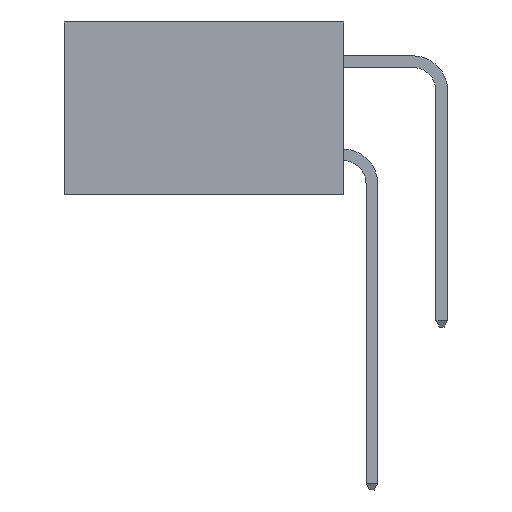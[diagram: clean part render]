
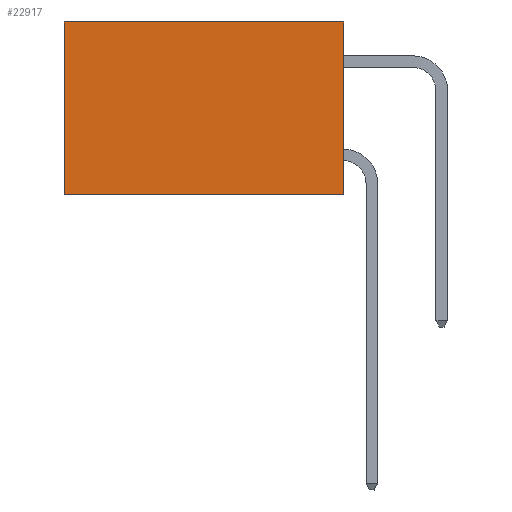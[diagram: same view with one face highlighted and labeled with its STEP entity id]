
A CAD part, left-side view. The second image highlights one B-rep face of the part: STEP entity #22917.
In plain terms, the highlighted planar face has unit normal (-1, 0, 0).
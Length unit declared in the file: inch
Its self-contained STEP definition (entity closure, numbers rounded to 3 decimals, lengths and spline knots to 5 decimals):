
#983 = VECTOR ( 'NONE', #11977, 39.37008 ) ;
#1222 = VERTEX_POINT ( 'NONE', #29377 ) ;
#1296 = VERTEX_POINT ( 'NONE', #10674 ) ;
#2550 = DIRECTION ( 'NONE',  ( 0., 0., -1. ) ) ;
#4002 = LINE ( 'NONE', #14784, #24245 ) ;
#4293 = ORIENTED_EDGE ( 'NONE', *, *, #30141, .T. ) ;
#5652 = DIRECTION ( 'NONE',  ( 0., 1., 0. ) ) ;
#5826 = VECTOR ( 'NONE', #16927, 39.37008 ) ;
#6339 = VERTEX_POINT ( 'NONE', #23426 ) ;
#6565 = ORIENTED_EDGE ( 'NONE', *, *, #25584, .F. ) ;
#8613 = AXIS2_PLACEMENT_3D ( 'NONE', #11788, #23866, #2550 ) ;
#9374 = EDGE_LOOP ( 'NONE', ( #15632, #6565, #12265, #4293 ) ) ;
#9980 = LINE ( 'NONE', #26327, #983 ) ;
#10674 = CARTESIAN_POINT ( 'NONE',  ( 0.298, 0.6, -0.37 ) ) ;
#11370 = EDGE_CURVE ( 'NONE', #1222, #6339, #28977, .T. ) ;
#11788 = CARTESIAN_POINT ( 'NONE',  ( 0.298, 0., 0. ) ) ;
#11977 = DIRECTION ( 'NONE',  ( 0., 1., 0. ) ) ;
#12265 = ORIENTED_EDGE ( 'NONE', *, *, #11370, .F. ) ;
#13321 = CARTESIAN_POINT ( 'NONE',  ( 0.298, 0., -0.37 ) ) ;
#14045 = VERTEX_POINT ( 'NONE', #15952 ) ;
#14784 = CARTESIAN_POINT ( 'NONE',  ( 0.298, 0.6, 0. ) ) ;
#15446 = FACE_OUTER_BOUND ( 'NONE', #9374, .T. ) ;
#15632 = ORIENTED_EDGE ( 'NONE', *, *, #17212, .T. ) ;
#15952 = CARTESIAN_POINT ( 'NONE',  ( 0.298, 0.6, 0. ) ) ;
#16927 = DIRECTION ( 'NONE',  ( 0., 0., -1. ) ) ;
#17212 = EDGE_CURVE ( 'NONE', #14045, #1296, #4002, .T. ) ;
#18742 = PLANE ( 'NONE',  #8613 ) ;
#19406 = VECTOR ( 'NONE', #5652, 39.37008 ) ;
#22917 = ADVANCED_FACE ( 'NONE', ( #15446 ), #18742, .F. ) ;
#23426 = CARTESIAN_POINT ( 'NONE',  ( 0.298, 0., -0.37 ) ) ;
#23508 = LINE ( 'NONE', #13321, #19406 ) ;
#23866 = DIRECTION ( 'NONE',  ( 1., 0., 0. ) ) ;
#24245 = VECTOR ( 'NONE', #29925, 39.37008 ) ;
#25584 = EDGE_CURVE ( 'NONE', #6339, #1296, #23508, .T. ) ;
#26327 = CARTESIAN_POINT ( 'NONE',  ( 0.298, 0., 0. ) ) ;
#28271 = CARTESIAN_POINT ( 'NONE',  ( 0.298, 0., 0. ) ) ;
#28977 = LINE ( 'NONE', #28271, #5826 ) ;
#29377 = CARTESIAN_POINT ( 'NONE',  ( 0.298, 0., 0. ) ) ;
#29925 = DIRECTION ( 'NONE',  ( 0., 0., -1. ) ) ;
#30141 = EDGE_CURVE ( 'NONE', #1222, #14045, #9980, .T. ) ;
